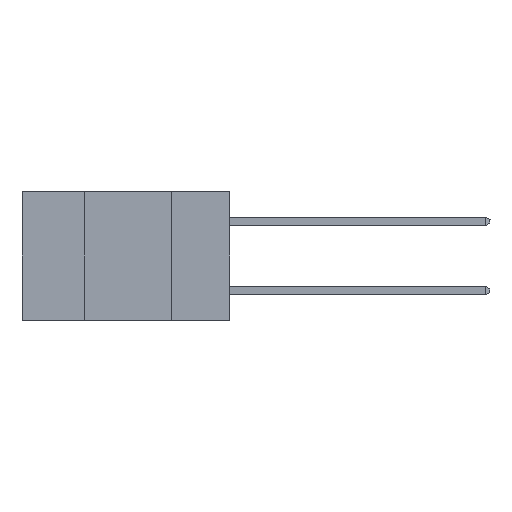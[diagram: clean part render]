
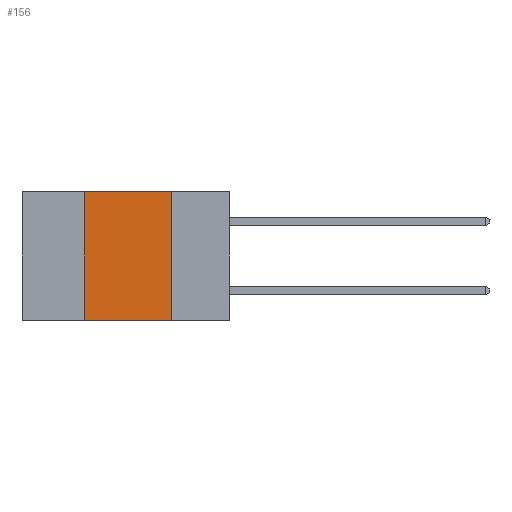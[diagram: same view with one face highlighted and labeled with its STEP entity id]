
A CAD part, left-side view. The second image highlights one B-rep face of the part: STEP entity #156.
In plain terms, the highlighted planar face has unit normal (-1, 0, 0).
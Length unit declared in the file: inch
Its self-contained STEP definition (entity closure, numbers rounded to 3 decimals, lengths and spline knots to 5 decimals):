
#156 = ADVANCED_FACE ( 'NONE', ( #4936 ), #6827, .F. ) ;
#243 = DIRECTION ( 'NONE',  ( 0., 0., -1. ) ) ;
#619 = LINE ( 'NONE', #6688, #6333 ) ;
#865 = CARTESIAN_POINT ( 'NONE',  ( 0., 0.6, -0.37 ) ) ;
#1572 = CARTESIAN_POINT ( 'NONE',  ( 0., 0.6, 0. ) ) ;
#1812 = CARTESIAN_POINT ( 'NONE',  ( 0., 0.42, 0. ) ) ;
#3343 = LINE ( 'NONE', #6361, #12772 ) ;
#3393 = DIRECTION ( 'NONE',  ( 1., 0., 0. ) ) ;
#3708 = EDGE_LOOP ( 'NONE', ( #18577, #16277, #17800, #9516 ) ) ;
#4152 = VERTEX_POINT ( 'NONE', #1812 ) ;
#4674 = VERTEX_POINT ( 'NONE', #9757 ) ;
#4936 = FACE_OUTER_BOUND ( 'NONE', #3708, .T. ) ;
#5654 = LINE ( 'NONE', #865, #6341 ) ;
#6333 = VECTOR ( 'NONE', #16496, 39.37008 ) ;
#6341 = VECTOR ( 'NONE', #14870, 39.37008 ) ;
#6361 = CARTESIAN_POINT ( 'NONE',  ( 0., 0.17, -0.37 ) ) ;
#6688 = CARTESIAN_POINT ( 'NONE',  ( 0., 0.42, -0.37 ) ) ;
#6827 = PLANE ( 'NONE',  #20221 ) ;
#8221 = EDGE_CURVE ( 'NONE', #4152, #4674, #17562, .T. ) ;
#8370 = EDGE_CURVE ( 'NONE', #19085, #4152, #619, .T. ) ;
#9516 = ORIENTED_EDGE ( 'NONE', *, *, #17812, .T. ) ;
#9757 = CARTESIAN_POINT ( 'NONE',  ( 0., 0.17, 0. ) ) ;
#12772 = VECTOR ( 'NONE', #14415, 39.37008 ) ;
#13208 = EDGE_CURVE ( 'NONE', #4674, #19591, #3343, .T. ) ;
#13380 = CARTESIAN_POINT ( 'NONE',  ( 0., 0.17, -0.37 ) ) ;
#14415 = DIRECTION ( 'NONE',  ( 0., 0., -1. ) ) ;
#14870 = DIRECTION ( 'NONE',  ( 0., -1., 0. ) ) ;
#15924 = CARTESIAN_POINT ( 'NONE',  ( 0., 0.6, 0. ) ) ;
#16277 = ORIENTED_EDGE ( 'NONE', *, *, #8221, .F. ) ;
#16496 = DIRECTION ( 'NONE',  ( 0., 0., 1. ) ) ;
#17562 = LINE ( 'NONE', #1572, #18684 ) ;
#17800 = ORIENTED_EDGE ( 'NONE', *, *, #8370, .F. ) ;
#17812 = EDGE_CURVE ( 'NONE', #19085, #19591, #5654, .T. ) ;
#17814 = CARTESIAN_POINT ( 'NONE',  ( 0., 0.42, -0.37 ) ) ;
#18577 = ORIENTED_EDGE ( 'NONE', *, *, #13208, .F. ) ;
#18684 = VECTOR ( 'NONE', #18810, 39.37008 ) ;
#18810 = DIRECTION ( 'NONE',  ( 0., -1., 0. ) ) ;
#19085 = VERTEX_POINT ( 'NONE', #17814 ) ;
#19591 = VERTEX_POINT ( 'NONE', #13380 ) ;
#20221 = AXIS2_PLACEMENT_3D ( 'NONE', #15924, #3393, #243 ) ;
